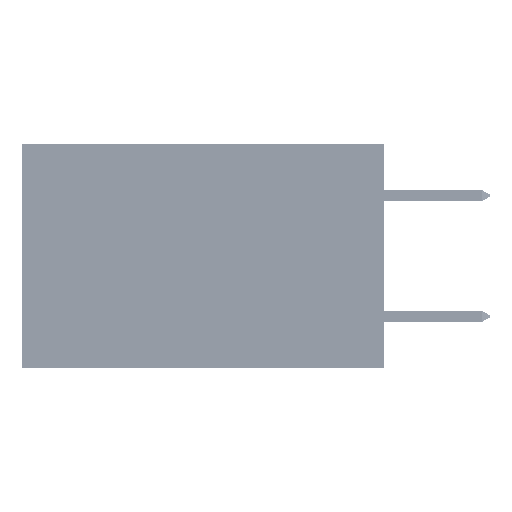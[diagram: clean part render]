
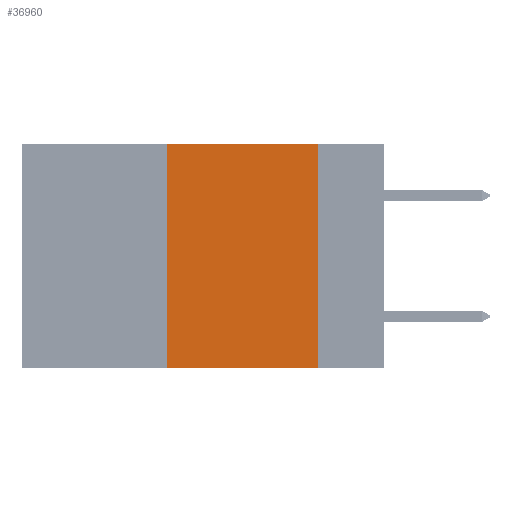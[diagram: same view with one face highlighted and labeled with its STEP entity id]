
A CAD part, left-side view. The second image highlights one B-rep face of the part: STEP entity #36960.
In plain terms, the highlighted planar face has unit normal (-1, 0, 0).
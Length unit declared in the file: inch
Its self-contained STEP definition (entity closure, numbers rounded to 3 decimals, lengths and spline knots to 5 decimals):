
#508 = ORIENTED_EDGE ( 'NONE', *, *, #41960, .F. ) ;
#1428 = CARTESIAN_POINT ( 'NONE',  ( 0., 0.6, -0.37 ) ) ;
#3145 = LINE ( 'NONE', #49232, #49769 ) ;
#4420 = VERTEX_POINT ( 'NONE', #26881 ) ;
#5614 = DIRECTION ( 'NONE',  ( 0., 0., 1. ) ) ;
#7634 = VERTEX_POINT ( 'NONE', #40254 ) ;
#9093 = LINE ( 'NONE', #10802, #51354 ) ;
#9660 = EDGE_CURVE ( 'NONE', #35211, #7634, #26487, .T. ) ;
#10166 = DIRECTION ( 'NONE',  ( 0., -1., 0. ) ) ;
#10519 = CARTESIAN_POINT ( 'NONE',  ( 0., 0.6, 0. ) ) ;
#10802 = CARTESIAN_POINT ( 'NONE',  ( 0., 0.11, 0. ) ) ;
#15055 = DIRECTION ( 'NONE',  ( 1., 0., 0. ) ) ;
#19510 = LINE ( 'NONE', #1428, #49998 ) ;
#21972 = ORIENTED_EDGE ( 'NONE', *, *, #27912, .T. ) ;
#23603 = DIRECTION ( 'NONE',  ( 0., 0., -1. ) ) ;
#25473 = AXIS2_PLACEMENT_3D ( 'NONE', #27601, #15055, #23603 ) ;
#26487 = LINE ( 'NONE', #10519, #43211 ) ;
#26881 = CARTESIAN_POINT ( 'NONE',  ( 0., 0.11, -0.37 ) ) ;
#27052 = CARTESIAN_POINT ( 'NONE',  ( 0., 0.36, 0. ) ) ;
#27438 = PLANE ( 'NONE',  #25473 ) ;
#27601 = CARTESIAN_POINT ( 'NONE',  ( 0., 0.6, 0. ) ) ;
#27912 = EDGE_CURVE ( 'NONE', #29463, #4420, #19510, .T. ) ;
#28757 = FACE_OUTER_BOUND ( 'NONE', #41643, .T. ) ;
#29463 = VERTEX_POINT ( 'NONE', #46339 ) ;
#33673 = DIRECTION ( 'NONE',  ( 0., -1., 0. ) ) ;
#35211 = VERTEX_POINT ( 'NONE', #27052 ) ;
#36960 = ADVANCED_FACE ( 'NONE', ( #28757 ), #27438, .F. ) ;
#39062 = EDGE_CURVE ( 'NONE', #7634, #4420, #9093, .T. ) ;
#39657 = ORIENTED_EDGE ( 'NONE', *, *, #39062, .F. ) ;
#40254 = CARTESIAN_POINT ( 'NONE',  ( 0., 0.11, 0. ) ) ;
#40417 = ORIENTED_EDGE ( 'NONE', *, *, #9660, .F. ) ;
#41643 = EDGE_LOOP ( 'NONE', ( #39657, #40417, #508, #21972 ) ) ;
#41960 = EDGE_CURVE ( 'NONE', #29463, #35211, #3145, .T. ) ;
#43211 = VECTOR ( 'NONE', #10166, 39.37008 ) ;
#46339 = CARTESIAN_POINT ( 'NONE',  ( 0., 0.36, -0.37 ) ) ;
#46405 = DIRECTION ( 'NONE',  ( 0., 0., -1. ) ) ;
#49232 = CARTESIAN_POINT ( 'NONE',  ( 0., 0.36, 0. ) ) ;
#49769 = VECTOR ( 'NONE', #5614, 39.37008 ) ;
#49998 = VECTOR ( 'NONE', #33673, 39.37008 ) ;
#51354 = VECTOR ( 'NONE', #46405, 39.37008 ) ;
